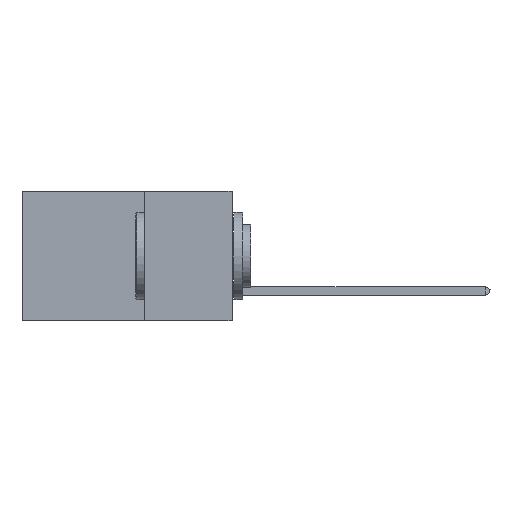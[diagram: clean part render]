
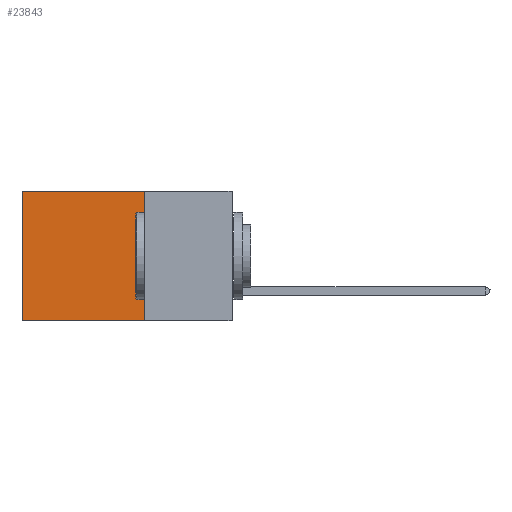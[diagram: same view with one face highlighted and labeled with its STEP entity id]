
A CAD part, left-side view. The second image highlights one B-rep face of the part: STEP entity #23843.
In plain terms, the highlighted planar face has unit normal (-1, 0, 0).
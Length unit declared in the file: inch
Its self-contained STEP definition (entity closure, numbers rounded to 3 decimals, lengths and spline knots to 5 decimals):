
#400 = CARTESIAN_POINT ( 'NONE',  ( 0.2875, 0.25, -0.37 ) ) ;
#604 = DIRECTION ( 'NONE',  ( 0., 1., 0. ) ) ;
#877 = CARTESIAN_POINT ( 'NONE',  ( 0.2875, 0.25, 0. ) ) ;
#1827 = LINE ( 'NONE', #15616, #21622 ) ;
#2262 = ORIENTED_EDGE ( 'NONE', *, *, #13085, .T. ) ;
#2337 = VECTOR ( 'NONE', #26882, 39.37008 ) ;
#3618 = DIRECTION ( 'NONE',  ( 1., 0., 0. ) ) ;
#6282 = PLANE ( 'NONE',  #25501 ) ;
#6356 = CARTESIAN_POINT ( 'NONE',  ( 0.2875, 0.25, 0. ) ) ;
#7641 = VERTEX_POINT ( 'NONE', #21410 ) ;
#9630 = LINE ( 'NONE', #24822, #18365 ) ;
#9746 = DIRECTION ( 'NONE',  ( 0., 0., -1. ) ) ;
#9762 = VERTEX_POINT ( 'NONE', #400 ) ;
#10952 = EDGE_CURVE ( 'NONE', #7641, #12174, #35089, .T. ) ;
#12061 = DIRECTION ( 'NONE',  ( 0., 0., -1. ) ) ;
#12174 = VERTEX_POINT ( 'NONE', #34842 ) ;
#13085 = EDGE_CURVE ( 'NONE', #12174, #28562, #9630, .T. ) ;
#15577 = CARTESIAN_POINT ( 'NONE',  ( 0.2875, 0.25, -0.37 ) ) ;
#15616 = CARTESIAN_POINT ( 'NONE',  ( 0.2875, 0.25, 0. ) ) ;
#15903 = ORIENTED_EDGE ( 'NONE', *, *, #16186, .F. ) ;
#16186 = EDGE_CURVE ( 'NONE', #9762, #28562, #35284, .T. ) ;
#18365 = VECTOR ( 'NONE', #27768, 39.37008 ) ;
#19166 = FACE_OUTER_BOUND ( 'NONE', #24052, .T. ) ;
#21410 = CARTESIAN_POINT ( 'NONE',  ( 0.2875, 0.25, 0. ) ) ;
#21622 = VECTOR ( 'NONE', #9746, 39.37008 ) ;
#23843 = ADVANCED_FACE ( 'NONE', ( #19166 ), #6282, .F. ) ;
#24052 = EDGE_LOOP ( 'NONE', ( #2262, #15903, #25607, #33754 ) ) ;
#24822 = CARTESIAN_POINT ( 'NONE',  ( 0.2875, 0.6, 0. ) ) ;
#25501 = AXIS2_PLACEMENT_3D ( 'NONE', #877, #3618, #12061 ) ;
#25607 = ORIENTED_EDGE ( 'NONE', *, *, #33033, .F. ) ;
#26882 = DIRECTION ( 'NONE',  ( 0., 1., 0. ) ) ;
#27768 = DIRECTION ( 'NONE',  ( 0., 0., -1. ) ) ;
#28562 = VERTEX_POINT ( 'NONE', #30422 ) ;
#30422 = CARTESIAN_POINT ( 'NONE',  ( 0.2875, 0.6, -0.37 ) ) ;
#31132 = VECTOR ( 'NONE', #604, 39.37008 ) ;
#33033 = EDGE_CURVE ( 'NONE', #7641, #9762, #1827, .T. ) ;
#33754 = ORIENTED_EDGE ( 'NONE', *, *, #10952, .T. ) ;
#34842 = CARTESIAN_POINT ( 'NONE',  ( 0.2875, 0.6, 0. ) ) ;
#35089 = LINE ( 'NONE', #6356, #31132 ) ;
#35284 = LINE ( 'NONE', #15577, #2337 ) ;
